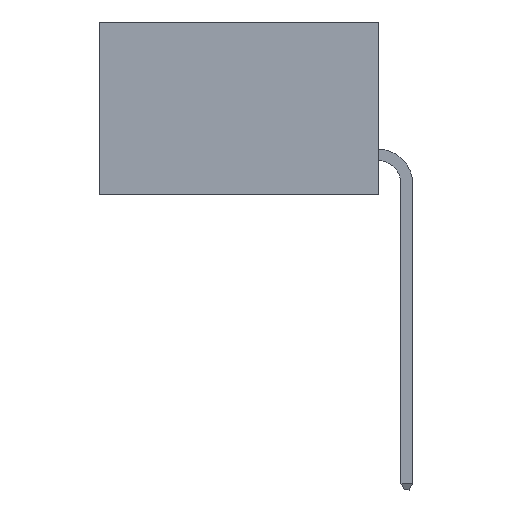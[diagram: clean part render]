
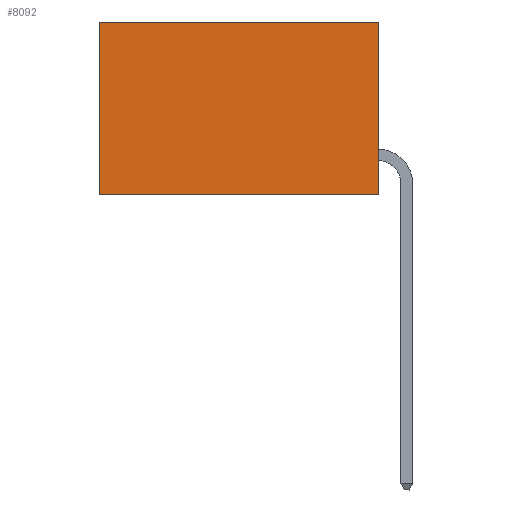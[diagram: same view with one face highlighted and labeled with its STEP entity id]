
A CAD part, left-side view. The second image highlights one B-rep face of the part: STEP entity #8092.
In plain terms, the highlighted planar face has unit normal (-1, 0, 0).
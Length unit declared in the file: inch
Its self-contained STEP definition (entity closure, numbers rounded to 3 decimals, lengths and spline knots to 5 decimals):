
#348 = EDGE_CURVE ( 'NONE', #4967, #3014, #3990, .T. ) ;
#350 = DIRECTION ( 'NONE',  ( 0., 0., -1. ) ) ;
#433 = AXIS2_PLACEMENT_3D ( 'NONE', #6596, #2350, #350 ) ;
#686 = EDGE_CURVE ( 'NONE', #2270, #4967, #5592, .T. ) ;
#1078 = EDGE_CURVE ( 'NONE', #2270, #3268, #7008, .T. ) ;
#1183 = ORIENTED_EDGE ( 'NONE', *, *, #686, .F. ) ;
#2002 = DIRECTION ( 'NONE',  ( 0., 0., -1. ) ) ;
#2270 = VERTEX_POINT ( 'NONE', #3482 ) ;
#2350 = DIRECTION ( 'NONE',  ( 1., 0., 0. ) ) ;
#2551 = CARTESIAN_POINT ( 'NONE',  ( 0.2615, 0., -0.37 ) ) ;
#3014 = VERTEX_POINT ( 'NONE', #5844 ) ;
#3210 = VECTOR ( 'NONE', #7609, 39.37008 ) ;
#3268 = VERTEX_POINT ( 'NONE', #5935 ) ;
#3482 = CARTESIAN_POINT ( 'NONE',  ( 0.2615, 0., 0. ) ) ;
#3990 = LINE ( 'NONE', #6825, #3210 ) ;
#4561 = VECTOR ( 'NONE', #8406, 39.37008 ) ;
#4601 = ORIENTED_EDGE ( 'NONE', *, *, #348, .F. ) ;
#4967 = VERTEX_POINT ( 'NONE', #2551 ) ;
#5125 = EDGE_CURVE ( 'NONE', #3268, #3014, #5727, .T. ) ;
#5219 = FACE_OUTER_BOUND ( 'NONE', #8036, .T. ) ;
#5592 = LINE ( 'NONE', #8216, #7593 ) ;
#5727 = LINE ( 'NONE', #9061, #8336 ) ;
#5844 = CARTESIAN_POINT ( 'NONE',  ( 0.2615, 0.6, -0.37 ) ) ;
#5935 = CARTESIAN_POINT ( 'NONE',  ( 0.2615, 0.6, 0. ) ) ;
#6368 = CARTESIAN_POINT ( 'NONE',  ( 0.2615, 0., 0. ) ) ;
#6596 = CARTESIAN_POINT ( 'NONE',  ( 0.2615, 0., -0.37 ) ) ;
#6825 = CARTESIAN_POINT ( 'NONE',  ( 0.2615, 0., -0.37 ) ) ;
#7008 = LINE ( 'NONE', #6368, #4561 ) ;
#7167 = ORIENTED_EDGE ( 'NONE', *, *, #1078, .T. ) ;
#7593 = VECTOR ( 'NONE', #2002, 39.37008 ) ;
#7609 = DIRECTION ( 'NONE',  ( 0., 1., 0. ) ) ;
#7890 = ORIENTED_EDGE ( 'NONE', *, *, #5125, .T. ) ;
#8036 = EDGE_LOOP ( 'NONE', ( #7890, #4601, #1183, #7167 ) ) ;
#8092 = ADVANCED_FACE ( 'NONE', ( #5219 ), #8650, .F. ) ;
#8216 = CARTESIAN_POINT ( 'NONE',  ( 0.2615, 0., -0.37 ) ) ;
#8336 = VECTOR ( 'NONE', #8375, 39.37008 ) ;
#8375 = DIRECTION ( 'NONE',  ( 0., 0., -1. ) ) ;
#8406 = DIRECTION ( 'NONE',  ( 0., 1., 0. ) ) ;
#8650 = PLANE ( 'NONE',  #433 ) ;
#9061 = CARTESIAN_POINT ( 'NONE',  ( 0.2615, 0.6, -0.37 ) ) ;
